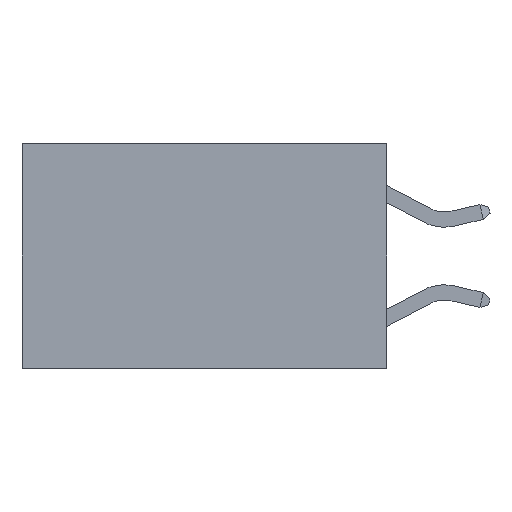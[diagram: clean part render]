
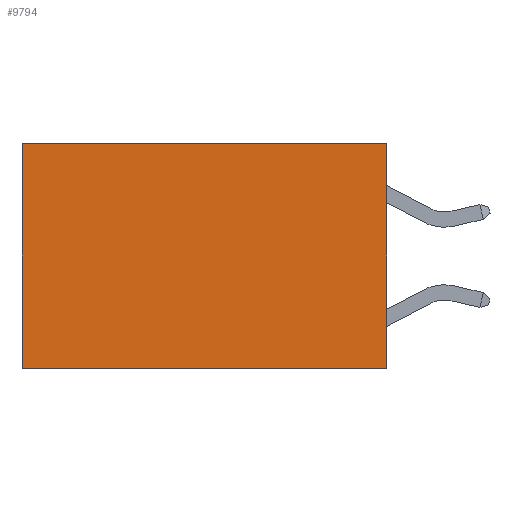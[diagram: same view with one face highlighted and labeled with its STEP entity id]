
A CAD part, left-side view. The second image highlights one B-rep face of the part: STEP entity #9794.
In plain terms, the highlighted planar face has unit normal (-1, 0, 0).
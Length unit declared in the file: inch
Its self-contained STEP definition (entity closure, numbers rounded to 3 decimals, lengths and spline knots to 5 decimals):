
#1231 = DIRECTION ( 'NONE',  ( 0., 0., -1. ) ) ;
#1296 = VECTOR ( 'NONE', #23674, 39.37008 ) ;
#1346 = VERTEX_POINT ( 'NONE', #9198 ) ;
#3153 = LINE ( 'NONE', #25090, #5076 ) ;
#3277 = PLANE ( 'NONE',  #19479 ) ;
#3501 = LINE ( 'NONE', #5259, #1296 ) ;
#3738 = CARTESIAN_POINT ( 'NONE',  ( 0.2625, 0., 0. ) ) ;
#4435 = EDGE_CURVE ( 'NONE', #13672, #5077, #18618, .T. ) ;
#5076 = VECTOR ( 'NONE', #6842, 39.37008 ) ;
#5077 = VERTEX_POINT ( 'NONE', #17294 ) ;
#5259 = CARTESIAN_POINT ( 'NONE',  ( 0.2625, 0., -0.37 ) ) ;
#5722 = DIRECTION ( 'NONE',  ( 0., 0., -1. ) ) ;
#6842 = DIRECTION ( 'NONE',  ( 0., 1., 0. ) ) ;
#9198 = CARTESIAN_POINT ( 'NONE',  ( 0.2625, 0.6, 0. ) ) ;
#9794 = ADVANCED_FACE ( 'NONE', ( #22460 ), #3277, .F. ) ;
#9840 = ORIENTED_EDGE ( 'NONE', *, *, #25111, .T. ) ;
#9882 = EDGE_CURVE ( 'NONE', #1346, #25424, #25614, .T. ) ;
#11476 = DIRECTION ( 'NONE',  ( 0., 0., -1. ) ) ;
#13672 = VERTEX_POINT ( 'NONE', #18984 ) ;
#15095 = VECTOR ( 'NONE', #5722, 39.37008 ) ;
#17294 = CARTESIAN_POINT ( 'NONE',  ( 0.2625, 0., -0.37 ) ) ;
#17570 = DIRECTION ( 'NONE',  ( 1., 0., 0. ) ) ;
#17730 = ORIENTED_EDGE ( 'NONE', *, *, #17825, .F. ) ;
#17825 = EDGE_CURVE ( 'NONE', #5077, #25424, #3501, .T. ) ;
#18618 = LINE ( 'NONE', #3738, #15095 ) ;
#18984 = CARTESIAN_POINT ( 'NONE',  ( 0.2625, 0., 0. ) ) ;
#19479 = AXIS2_PLACEMENT_3D ( 'NONE', #21295, #17570, #1231 ) ;
#19789 = CARTESIAN_POINT ( 'NONE',  ( 0.2625, 0.6, -0.37 ) ) ;
#19925 = VECTOR ( 'NONE', #11476, 39.37008 ) ;
#20209 = EDGE_LOOP ( 'NONE', ( #25795, #17730, #20257, #9840 ) ) ;
#20257 = ORIENTED_EDGE ( 'NONE', *, *, #4435, .F. ) ;
#21295 = CARTESIAN_POINT ( 'NONE',  ( 0.2625, 0., 0. ) ) ;
#22460 = FACE_OUTER_BOUND ( 'NONE', #20209, .T. ) ;
#23674 = DIRECTION ( 'NONE',  ( 0., 1., 0. ) ) ;
#25090 = CARTESIAN_POINT ( 'NONE',  ( 0.2625, 0., 0. ) ) ;
#25111 = EDGE_CURVE ( 'NONE', #13672, #1346, #3153, .T. ) ;
#25349 = CARTESIAN_POINT ( 'NONE',  ( 0.2625, 0.6, 0. ) ) ;
#25424 = VERTEX_POINT ( 'NONE', #19789 ) ;
#25614 = LINE ( 'NONE', #25349, #19925 ) ;
#25795 = ORIENTED_EDGE ( 'NONE', *, *, #9882, .T. ) ;
